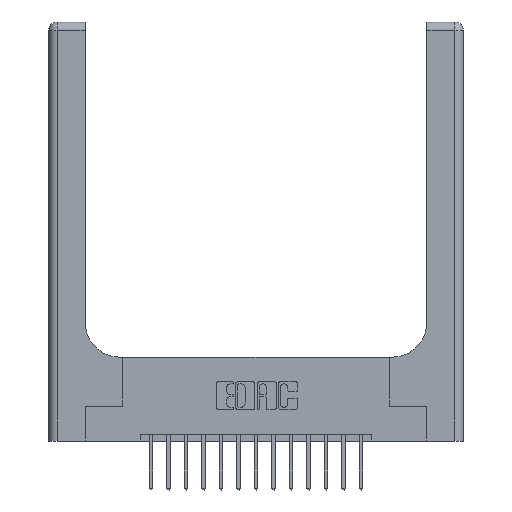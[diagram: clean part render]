
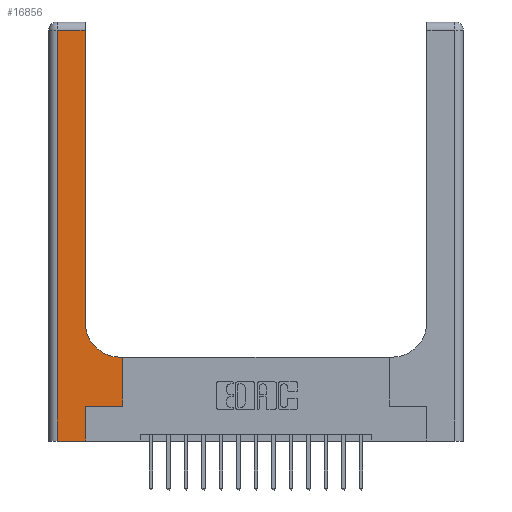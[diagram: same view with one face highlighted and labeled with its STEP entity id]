
A CAD part, top view. The second image highlights one B-rep face of the part: STEP entity #16856.
In plain terms, the highlighted planar face has unit normal (0, 0, 1).
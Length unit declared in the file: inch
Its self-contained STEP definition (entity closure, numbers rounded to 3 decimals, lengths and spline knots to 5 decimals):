
#228 = VERTEX_POINT ( 'NONE', #15237 ) ;
#243 = VECTOR ( 'NONE', #7607, 39.37008 ) ;
#375 = VERTEX_POINT ( 'NONE', #1821 ) ;
#400 = DIRECTION ( 'NONE',  ( -1., 0., 0. ) ) ;
#517 = VECTOR ( 'NONE', #7664, 39.37008 ) ;
#598 = CARTESIAN_POINT ( 'NONE',  ( 0.51, 0.6, 0.37 ) ) ;
#713 = VERTEX_POINT ( 'NONE', #17075 ) ;
#1620 = LINE ( 'NONE', #7212, #13920 ) ;
#1821 = CARTESIAN_POINT ( 'NONE',  ( 0.26, 0.85, 0.37 ) ) ;
#1887 = DIRECTION ( 'NONE',  ( 0., 1., 0. ) ) ;
#1977 = DIRECTION ( 'NONE',  ( 1., 0., 0. ) ) ;
#2020 = LINE ( 'NONE', #6320, #243 ) ;
#2206 = CARTESIAN_POINT ( 'NONE',  ( 0.265, 0.25, 0.37 ) ) ;
#2249 = CARTESIAN_POINT ( 'NONE',  ( 0., 0., 0.37 ) ) ;
#2661 = CARTESIAN_POINT ( 'NONE',  ( 0.265, 0., 0.37 ) ) ;
#2875 = DIRECTION ( 'NONE',  ( 0., 0., -1. ) ) ;
#2970 = PLANE ( 'NONE',  #13066 ) ;
#3354 = LINE ( 'NONE', #2249, #4912 ) ;
#3902 = CARTESIAN_POINT ( 'NONE',  ( 0.06, 3., 0.37 ) ) ;
#3954 = ORIENTED_EDGE ( 'NONE', *, *, #5548, .T. ) ;
#4173 = DIRECTION ( 'NONE',  ( 0., -1., 0. ) ) ;
#4258 = EDGE_CURVE ( 'NONE', #713, #14487, #3354, .T. ) ;
#4290 = EDGE_CURVE ( 'NONE', #375, #7497, #13356, .T. ) ;
#4912 = VECTOR ( 'NONE', #1977, 39.37008 ) ;
#5256 = ORIENTED_EDGE ( 'NONE', *, *, #17612, .T. ) ;
#5548 = EDGE_CURVE ( 'NONE', #16919, #713, #16310, .T. ) ;
#5623 = FACE_OUTER_BOUND ( 'NONE', #16739, .T. ) ;
#5808 = LINE ( 'NONE', #16940, #13936 ) ;
#6008 = ORIENTED_EDGE ( 'NONE', *, *, #7007, .T. ) ;
#6260 = EDGE_CURVE ( 'NONE', #9418, #16629, #2020, .T. ) ;
#6320 = CARTESIAN_POINT ( 'NONE',  ( 0.26, 0.6, 0.37 ) ) ;
#6429 = EDGE_CURVE ( 'NONE', #14487, #7528, #9342, .T. ) ;
#6449 = ORIENTED_EDGE ( 'NONE', *, *, #6429, .T. ) ;
#7007 = EDGE_CURVE ( 'NONE', #7497, #16919, #5808, .T. ) ;
#7212 = CARTESIAN_POINT ( 'NONE',  ( 0.265, 0.25, 0.37 ) ) ;
#7497 = VERTEX_POINT ( 'NONE', #9157 ) ;
#7528 = VERTEX_POINT ( 'NONE', #2206 ) ;
#7607 = DIRECTION ( 'NONE',  ( -1., 0., 0. ) ) ;
#7664 = DIRECTION ( 'NONE',  ( 0., 1., 0. ) ) ;
#7826 = DIRECTION ( 'NONE',  ( 1., 0., 0. ) ) ;
#8511 = VECTOR ( 'NONE', #4173, 39.37008 ) ;
#8838 = ORIENTED_EDGE ( 'NONE', *, *, #4258, .T. ) ;
#9157 = CARTESIAN_POINT ( 'NONE',  ( 0.26, 2.94, 0.37 ) ) ;
#9342 = LINE ( 'NONE', #2661, #16273 ) ;
#9418 = VERTEX_POINT ( 'NONE', #11117 ) ;
#10160 = ORIENTED_EDGE ( 'NONE', *, *, #4290, .T. ) ;
#10289 = ORIENTED_EDGE ( 'NONE', *, *, #14633, .T. ) ;
#11117 = CARTESIAN_POINT ( 'NONE',  ( 0.528, 0.6, 0.37 ) ) ;
#11162 = CARTESIAN_POINT ( 'NONE',  ( 0.06, 2.94, 0.37 ) ) ;
#11633 = CARTESIAN_POINT ( 'NONE',  ( 0.528, 0.25, 0.37 ) ) ;
#11803 = CARTESIAN_POINT ( 'NONE',  ( 0.265, 0., 0.37 ) ) ;
#12399 = DIRECTION ( 'NONE',  ( 0., 1., 0. ) ) ;
#12716 = CIRCLE ( 'NONE', #17985, 0.25 ) ;
#12805 = DIRECTION ( 'NONE',  ( -1., 0., 0. ) ) ;
#13066 = AXIS2_PLACEMENT_3D ( 'NONE', #14068, #2875, #400 ) ;
#13091 = VECTOR ( 'NONE', #1887, 39.37008 ) ;
#13356 = LINE ( 'NONE', #17309, #517 ) ;
#13443 = CARTESIAN_POINT ( 'NONE',  ( 0.51, 0.85, 0.37 ) ) ;
#13920 = VECTOR ( 'NONE', #7826, 39.37008 ) ;
#13936 = VECTOR ( 'NONE', #12805, 39.37008 ) ;
#14068 = CARTESIAN_POINT ( 'NONE',  ( 0., 3., 0.37 ) ) ;
#14365 = LINE ( 'NONE', #11633, #13091 ) ;
#14487 = VERTEX_POINT ( 'NONE', #11803 ) ;
#14633 = EDGE_CURVE ( 'NONE', #16629, #375, #12716, .T. ) ;
#15015 = ORIENTED_EDGE ( 'NONE', *, *, #6260, .T. ) ;
#15237 = CARTESIAN_POINT ( 'NONE',  ( 0.528, 0.25, 0.37 ) ) ;
#15483 = EDGE_CURVE ( 'NONE', #7528, #228, #1620, .T. ) ;
#15927 = ORIENTED_EDGE ( 'NONE', *, *, #15483, .T. ) ;
#16273 = VECTOR ( 'NONE', #12399, 39.37008 ) ;
#16303 = DIRECTION ( 'NONE',  ( 1., 0., 0. ) ) ;
#16310 = LINE ( 'NONE', #3902, #8511 ) ;
#16629 = VERTEX_POINT ( 'NONE', #598 ) ;
#16739 = EDGE_LOOP ( 'NONE', ( #10160, #6008, #3954, #8838, #6449, #15927, #5256, #15015, #10289 ) ) ;
#16856 = ADVANCED_FACE ( 'NONE', ( #5623 ), #2970, .F. ) ;
#16919 = VERTEX_POINT ( 'NONE', #11162 ) ;
#16940 = CARTESIAN_POINT ( 'NONE',  ( 0., 2.94, 0.37 ) ) ;
#17075 = CARTESIAN_POINT ( 'NONE',  ( 0.06, 0., 0.37 ) ) ;
#17309 = CARTESIAN_POINT ( 'NONE',  ( 0.26, 3., 0.37 ) ) ;
#17612 = EDGE_CURVE ( 'NONE', #228, #9418, #14365, .T. ) ;
#17651 = DIRECTION ( 'NONE',  ( 0., 0., -1. ) ) ;
#17985 = AXIS2_PLACEMENT_3D ( 'NONE', #13443, #17651, #16303 ) ;
